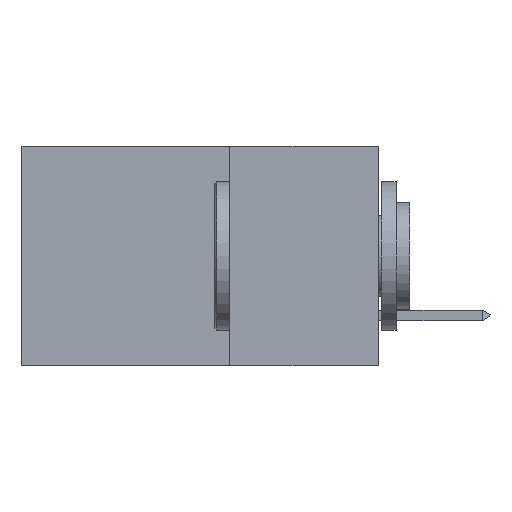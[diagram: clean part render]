
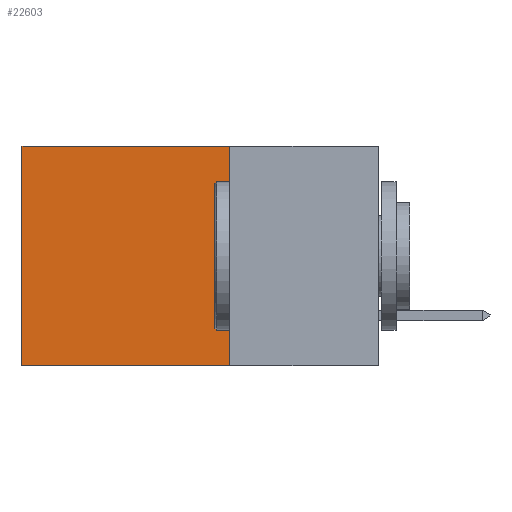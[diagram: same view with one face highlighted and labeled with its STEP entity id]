
A CAD part, left-side view. The second image highlights one B-rep face of the part: STEP entity #22603.
In plain terms, the highlighted planar face has unit normal (-1, 0, 0).
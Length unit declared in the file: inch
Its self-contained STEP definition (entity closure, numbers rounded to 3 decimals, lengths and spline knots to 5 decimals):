
#442 = VERTEX_POINT ( 'NONE', #21597 ) ;
#2456 = ORIENTED_EDGE ( 'NONE', *, *, #20766, .T. ) ;
#2719 = ORIENTED_EDGE ( 'NONE', *, *, #11825, .F. ) ;
#4500 = VERTEX_POINT ( 'NONE', #27302 ) ;
#5230 = ORIENTED_EDGE ( 'NONE', *, *, #8724, .T. ) ;
#5708 = VERTEX_POINT ( 'NONE', #17180 ) ;
#6569 = CARTESIAN_POINT ( 'NONE',  ( 0.298, 0.25, -0.37 ) ) ;
#8647 = CARTESIAN_POINT ( 'NONE',  ( 0.298, 0.25, 0. ) ) ;
#8724 = EDGE_CURVE ( 'NONE', #5708, #442, #8743, .T. ) ;
#8743 = LINE ( 'NONE', #27756, #15695 ) ;
#9598 = VECTOR ( 'NONE', #29849, 39.37008 ) ;
#11825 = EDGE_CURVE ( 'NONE', #27873, #4500, #29627, .T. ) ;
#12543 = CARTESIAN_POINT ( 'NONE',  ( 0.298, 0.6, 0. ) ) ;
#13555 = DIRECTION ( 'NONE',  ( 0., 0., -1. ) ) ;
#13869 = LINE ( 'NONE', #12543, #26966 ) ;
#14165 = LINE ( 'NONE', #29652, #29443 ) ;
#15541 = DIRECTION ( 'NONE',  ( 0., 0., -1. ) ) ;
#15695 = VECTOR ( 'NONE', #20865, 39.37008 ) ;
#17180 = CARTESIAN_POINT ( 'NONE',  ( 0.298, 0.25, 0. ) ) ;
#19062 = AXIS2_PLACEMENT_3D ( 'NONE', #8647, #25164, #13555 ) ;
#19555 = FACE_OUTER_BOUND ( 'NONE', #24672, .T. ) ;
#20095 = CARTESIAN_POINT ( 'NONE',  ( 0.298, 0.25, -0.37 ) ) ;
#20546 = ORIENTED_EDGE ( 'NONE', *, *, #21578, .F. ) ;
#20766 = EDGE_CURVE ( 'NONE', #442, #4500, #13869, .T. ) ;
#20865 = DIRECTION ( 'NONE',  ( 0., 1., 0. ) ) ;
#21578 = EDGE_CURVE ( 'NONE', #5708, #27873, #14165, .T. ) ;
#21597 = CARTESIAN_POINT ( 'NONE',  ( 0.298, 0.6, 0. ) ) ;
#22603 = ADVANCED_FACE ( 'NONE', ( #19555 ), #22856, .F. ) ;
#22856 = PLANE ( 'NONE',  #19062 ) ;
#24672 = EDGE_LOOP ( 'NONE', ( #2456, #2719, #20546, #5230 ) ) ;
#25164 = DIRECTION ( 'NONE',  ( 1., 0., 0. ) ) ;
#26583 = DIRECTION ( 'NONE',  ( 0., 0., -1. ) ) ;
#26966 = VECTOR ( 'NONE', #26583, 39.37008 ) ;
#27302 = CARTESIAN_POINT ( 'NONE',  ( 0.298, 0.6, -0.37 ) ) ;
#27756 = CARTESIAN_POINT ( 'NONE',  ( 0.298, 0.25, 0. ) ) ;
#27873 = VERTEX_POINT ( 'NONE', #20095 ) ;
#29443 = VECTOR ( 'NONE', #15541, 39.37008 ) ;
#29627 = LINE ( 'NONE', #6569, #9598 ) ;
#29652 = CARTESIAN_POINT ( 'NONE',  ( 0.298, 0.25, 0. ) ) ;
#29849 = DIRECTION ( 'NONE',  ( 0., 1., 0. ) ) ;
